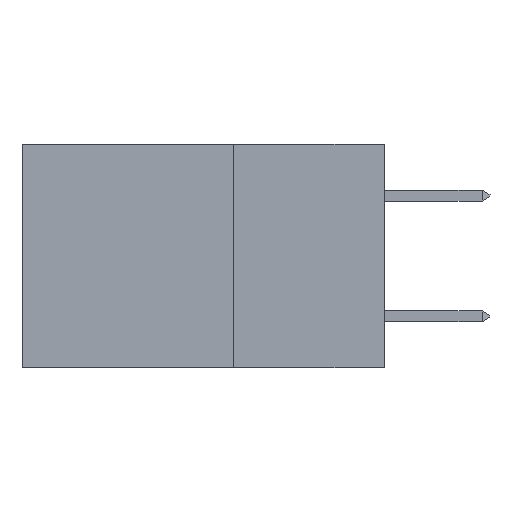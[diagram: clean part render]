
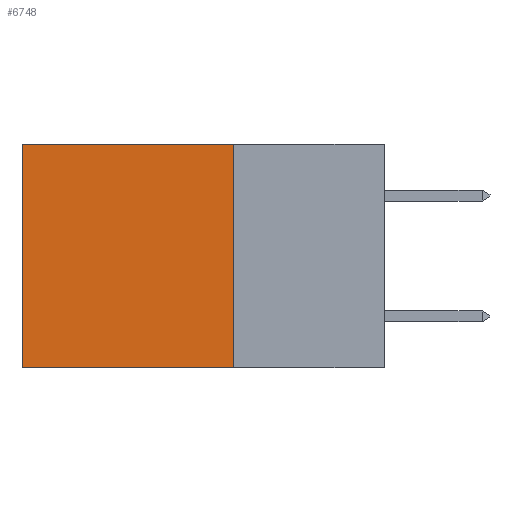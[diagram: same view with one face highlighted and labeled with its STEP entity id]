
A CAD part, left-side view. The second image highlights one B-rep face of the part: STEP entity #6748.
In plain terms, the highlighted planar face has unit normal (-1, 0, 0).
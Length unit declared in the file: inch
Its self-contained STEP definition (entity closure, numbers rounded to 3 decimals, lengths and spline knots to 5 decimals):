
#521 = VERTEX_POINT ( 'NONE', #15702 ) ;
#583 = EDGE_CURVE ( 'NONE', #7825, #13574, #1093, .T. ) ;
#1063 = CARTESIAN_POINT ( 'NONE',  ( 0.2875, 0.25, -0.37 ) ) ;
#1093 = LINE ( 'NONE', #13888, #10852 ) ;
#1825 = VERTEX_POINT ( 'NONE', #6862 ) ;
#2551 = ORIENTED_EDGE ( 'NONE', *, *, #3387, .F. ) ;
#3075 = EDGE_CURVE ( 'NONE', #521, #13574, #15638, .T. ) ;
#3105 = AXIS2_PLACEMENT_3D ( 'NONE', #4540, #4380, #4345 ) ;
#3387 = EDGE_CURVE ( 'NONE', #1825, #7825, #11375, .T. ) ;
#3459 = ORIENTED_EDGE ( 'NONE', *, *, #4459, .T. ) ;
#4023 = DIRECTION ( 'NONE',  ( 0., 0., -1. ) ) ;
#4257 = CARTESIAN_POINT ( 'NONE',  ( 0.2875, 0.25, 0. ) ) ;
#4345 = DIRECTION ( 'NONE',  ( 0., 0., -1. ) ) ;
#4380 = DIRECTION ( 'NONE',  ( 1., 0., 0. ) ) ;
#4433 = PLANE ( 'NONE',  #3105 ) ;
#4459 = EDGE_CURVE ( 'NONE', #1825, #521, #7961, .T. ) ;
#4540 = CARTESIAN_POINT ( 'NONE',  ( 0.2875, 0.25, 0. ) ) ;
#6634 = EDGE_LOOP ( 'NONE', ( #9921, #7110, #2551, #3459 ) ) ;
#6748 = ADVANCED_FACE ( 'NONE', ( #9291 ), #4433, .F. ) ;
#6862 = CARTESIAN_POINT ( 'NONE',  ( 0.2875, 0.25, 0. ) ) ;
#7110 = ORIENTED_EDGE ( 'NONE', *, *, #583, .F. ) ;
#7557 = VECTOR ( 'NONE', #8537, 39.37008 ) ;
#7825 = VERTEX_POINT ( 'NONE', #1063 ) ;
#7961 = LINE ( 'NONE', #8569, #7557 ) ;
#8036 = VECTOR ( 'NONE', #4023, 39.37008 ) ;
#8537 = DIRECTION ( 'NONE',  ( 0., 1., 0. ) ) ;
#8569 = CARTESIAN_POINT ( 'NONE',  ( 0.2875, 0.25, 0. ) ) ;
#9234 = VECTOR ( 'NONE', #11204, 39.37008 ) ;
#9291 = FACE_OUTER_BOUND ( 'NONE', #6634, .T. ) ;
#9908 = CARTESIAN_POINT ( 'NONE',  ( 0.2875, 0.6, -0.37 ) ) ;
#9921 = ORIENTED_EDGE ( 'NONE', *, *, #3075, .T. ) ;
#10852 = VECTOR ( 'NONE', #15262, 39.37008 ) ;
#11183 = CARTESIAN_POINT ( 'NONE',  ( 0.2875, 0.6, 0. ) ) ;
#11204 = DIRECTION ( 'NONE',  ( 0., 0., -1. ) ) ;
#11375 = LINE ( 'NONE', #4257, #8036 ) ;
#13574 = VERTEX_POINT ( 'NONE', #9908 ) ;
#13888 = CARTESIAN_POINT ( 'NONE',  ( 0.2875, 0.25, -0.37 ) ) ;
#15262 = DIRECTION ( 'NONE',  ( 0., 1., 0. ) ) ;
#15638 = LINE ( 'NONE', #11183, #9234 ) ;
#15702 = CARTESIAN_POINT ( 'NONE',  ( 0.2875, 0.6, 0. ) ) ;
